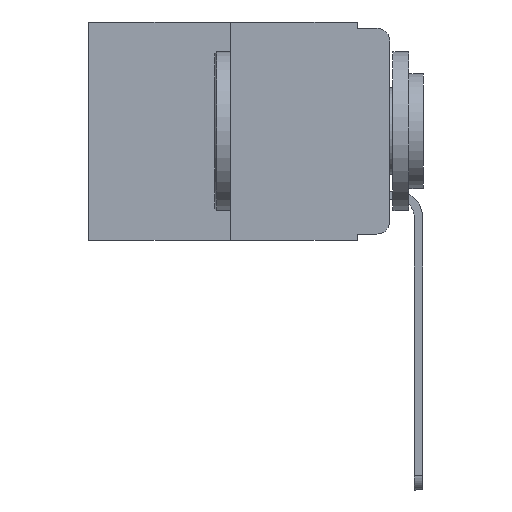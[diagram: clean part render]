
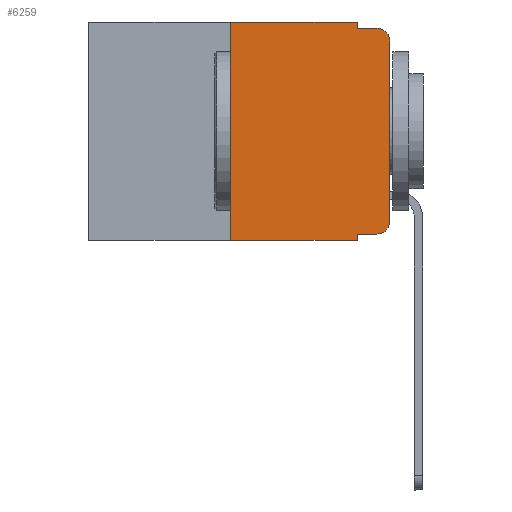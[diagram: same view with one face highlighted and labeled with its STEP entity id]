
A CAD part, left-side view. The second image highlights one B-rep face of the part: STEP entity #6259.
In plain terms, the highlighted planar face has unit normal (-1, 0, 0).
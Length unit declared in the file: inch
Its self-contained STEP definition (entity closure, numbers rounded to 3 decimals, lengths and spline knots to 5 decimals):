
#74 = CARTESIAN_POINT ( 'NONE',  ( 0., 0.051, 0. ) ) ;
#261 = CARTESIAN_POINT ( 'NONE',  ( 0., 0.25, 0. ) ) ;
#341 = LINE ( 'NONE', #1456, #7320 ) ;
#374 = CARTESIAN_POINT ( 'NONE',  ( 0., 0.473, -0.343 ) ) ;
#627 = LINE ( 'NONE', #5079, #11566 ) ;
#925 = VECTOR ( 'NONE', #10586, 39.37008 ) ;
#939 = CARTESIAN_POINT ( 'NONE',  ( 0., 0.051, 0. ) ) ;
#945 = VERTEX_POINT ( 'NONE', #11992 ) ;
#1030 = LINE ( 'NONE', #74, #9752 ) ;
#1456 = CARTESIAN_POINT ( 'NONE',  ( 0., 0.473, 0. ) ) ;
#1624 = ORIENTED_EDGE ( 'NONE', *, *, #3747, .T. ) ;
#1734 = DIRECTION ( 'NONE',  ( 0., 0., 1. ) ) ;
#1830 = DIRECTION ( 'NONE',  ( 0., 0., -1. ) ) ;
#2245 = ORIENTED_EDGE ( 'NONE', *, *, #7513, .T. ) ;
#2343 = VERTEX_POINT ( 'NONE', #5365 ) ;
#2590 = VECTOR ( 'NONE', #9396, 39.37008 ) ;
#2623 = CARTESIAN_POINT ( 'NONE',  ( 0., 0.051, -0.343 ) ) ;
#2650 = VECTOR ( 'NONE', #2709, 39.37008 ) ;
#2709 = DIRECTION ( 'NONE',  ( 0., 0., -1. ) ) ;
#2778 = EDGE_CURVE ( 'NONE', #13716, #2343, #1030, .T. ) ;
#2904 = DIRECTION ( 'NONE',  ( -1., 0., 0. ) ) ;
#2912 = VERTEX_POINT ( 'NONE', #13113 ) ;
#3055 = VERTEX_POINT ( 'NONE', #3337 ) ;
#3180 = ORIENTED_EDGE ( 'NONE', *, *, #5538, .T. ) ;
#3337 = CARTESIAN_POINT ( 'NONE',  ( 0., 0.25, -0.343 ) ) ;
#3747 = EDGE_CURVE ( 'NONE', #3055, #5438, #10519, .T. ) ;
#3881 = LINE ( 'NONE', #14028, #2650 ) ;
#4073 = ORIENTED_EDGE ( 'NONE', *, *, #5902, .F. ) ;
#4097 = CARTESIAN_POINT ( 'NONE',  ( 0., 0.473, 0. ) ) ;
#4137 = CARTESIAN_POINT ( 'NONE',  ( 0., 0.02, -0.333 ) ) ;
#4330 = DIRECTION ( 'NONE',  ( 0., -1., 0. ) ) ;
#4398 = ORIENTED_EDGE ( 'NONE', *, *, #8779, .F. ) ;
#4459 = DIRECTION ( 'NONE',  ( 0., 0., -1. ) ) ;
#4486 = VERTEX_POINT ( 'NONE', #261 ) ;
#4524 = DIRECTION ( 'NONE',  ( 0., -1., 0. ) ) ;
#4825 = ORIENTED_EDGE ( 'NONE', *, *, #7428, .F. ) ;
#4941 = CARTESIAN_POINT ( 'NONE',  ( 0., 0., 0. ) ) ;
#4953 = EDGE_CURVE ( 'NONE', #7884, #5438, #3881, .T. ) ;
#5079 = CARTESIAN_POINT ( 'NONE',  ( 0., 0.25, 0. ) ) ;
#5342 = LINE ( 'NONE', #10810, #10851 ) ;
#5365 = CARTESIAN_POINT ( 'NONE',  ( 0., 0.051, -0.01 ) ) ;
#5406 = DIRECTION ( 'NONE',  ( 0., 0., -1. ) ) ;
#5438 = VERTEX_POINT ( 'NONE', #2623 ) ;
#5538 = EDGE_CURVE ( 'NONE', #945, #11118, #13760, .T. ) ;
#5756 = ORIENTED_EDGE ( 'NONE', *, *, #5799, .T. ) ;
#5799 = EDGE_CURVE ( 'NONE', #11933, #2912, #8650, .T. ) ;
#5863 = AXIS2_PLACEMENT_3D ( 'NONE', #4097, #9371, #13893 ) ;
#5902 = EDGE_CURVE ( 'NONE', #2343, #11118, #12829, .T. ) ;
#5958 = LINE ( 'NONE', #4941, #13860 ) ;
#6259 = ADVANCED_FACE ( 'NONE', ( #7379 ), #10809, .F. ) ;
#6261 = CARTESIAN_POINT ( 'NONE',  ( 0., 0.02, -0.03 ) ) ;
#6436 = ORIENTED_EDGE ( 'NONE', *, *, #11100, .T. ) ;
#6542 = AXIS2_PLACEMENT_3D ( 'NONE', #8917, #9188, #4459 ) ;
#7320 = VECTOR ( 'NONE', #4524, 39.37008 ) ;
#7379 = FACE_OUTER_BOUND ( 'NONE', #12621, .T. ) ;
#7428 = EDGE_CURVE ( 'NONE', #4486, #13716, #341, .T. ) ;
#7513 = EDGE_CURVE ( 'NONE', #2912, #945, #5958, .T. ) ;
#7884 = VERTEX_POINT ( 'NONE', #11499 ) ;
#8650 = CIRCLE ( 'NONE', #6542, 0.02 ) ;
#8779 = EDGE_CURVE ( 'NONE', #3055, #4486, #627, .T. ) ;
#8917 = CARTESIAN_POINT ( 'NONE',  ( 0., 0.02, -0.313 ) ) ;
#9188 = DIRECTION ( 'NONE',  ( -1., 0., 0. ) ) ;
#9262 = CARTESIAN_POINT ( 'NONE',  ( 0., 0.051, -0.01 ) ) ;
#9371 = DIRECTION ( 'NONE',  ( 1., 0., 0. ) ) ;
#9396 = DIRECTION ( 'NONE',  ( 0., -1., 0. ) ) ;
#9752 = VECTOR ( 'NONE', #5406, 39.37008 ) ;
#10519 = LINE ( 'NONE', #374, #925 ) ;
#10586 = DIRECTION ( 'NONE',  ( 0., -1., 0. ) ) ;
#10809 = PLANE ( 'NONE',  #5863 ) ;
#10810 = CARTESIAN_POINT ( 'NONE',  ( 0., 0.051, -0.333 ) ) ;
#10851 = VECTOR ( 'NONE', #4330, 39.37008 ) ;
#11100 = EDGE_CURVE ( 'NONE', #7884, #11933, #5342, .T. ) ;
#11118 = VERTEX_POINT ( 'NONE', #13234 ) ;
#11499 = CARTESIAN_POINT ( 'NONE',  ( 0., 0.051, -0.333 ) ) ;
#11566 = VECTOR ( 'NONE', #1734, 39.37008 ) ;
#11894 = AXIS2_PLACEMENT_3D ( 'NONE', #6261, #2904, #1830 ) ;
#11933 = VERTEX_POINT ( 'NONE', #4137 ) ;
#11992 = CARTESIAN_POINT ( 'NONE',  ( 0., 0., -0.03 ) ) ;
#12564 = ORIENTED_EDGE ( 'NONE', *, *, #4953, .F. ) ;
#12621 = EDGE_LOOP ( 'NONE', ( #2245, #3180, #4073, #13181, #4825, #4398, #1624, #12564, #6436, #5756 ) ) ;
#12829 = LINE ( 'NONE', #9262, #2590 ) ;
#13113 = CARTESIAN_POINT ( 'NONE',  ( 0., 0., -0.313 ) ) ;
#13181 = ORIENTED_EDGE ( 'NONE', *, *, #2778, .F. ) ;
#13234 = CARTESIAN_POINT ( 'NONE',  ( 0., 0.02, -0.01 ) ) ;
#13716 = VERTEX_POINT ( 'NONE', #939 ) ;
#13760 = CIRCLE ( 'NONE', #11894, 0.02 ) ;
#13860 = VECTOR ( 'NONE', #14063, 39.37008 ) ;
#13893 = DIRECTION ( 'NONE',  ( 0., 0., -1. ) ) ;
#14028 = CARTESIAN_POINT ( 'NONE',  ( 0., 0.051, 0. ) ) ;
#14063 = DIRECTION ( 'NONE',  ( 0., 0., 1. ) ) ;
